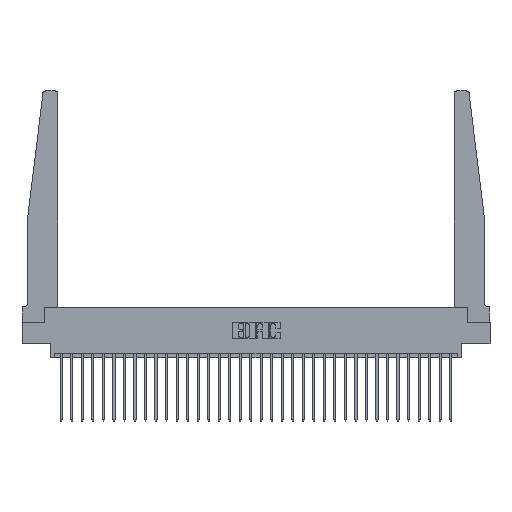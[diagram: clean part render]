
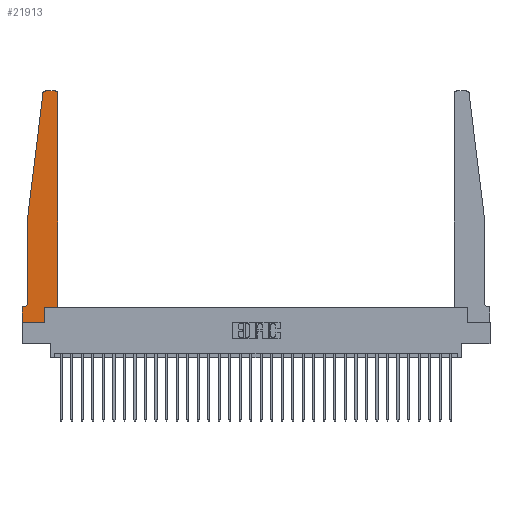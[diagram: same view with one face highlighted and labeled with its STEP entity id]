
A CAD part, top view. The second image highlights one B-rep face of the part: STEP entity #21913.
In plain terms, the highlighted planar face has unit normal (0, 0, 1).
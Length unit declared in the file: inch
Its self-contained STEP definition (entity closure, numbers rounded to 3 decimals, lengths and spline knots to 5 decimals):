
#366 = VERTEX_POINT ( 'NONE', #1723 ) ;
#1034 = CARTESIAN_POINT ( 'NONE',  ( 0., 0.1875, 0.37 ) ) ;
#1373 = CARTESIAN_POINT ( 'NONE',  ( 0.065, 1.25, 0.37 ) ) ;
#1605 = CIRCLE ( 'NONE', #3086, 0.03 ) ;
#1723 = CARTESIAN_POINT ( 'NONE',  ( 0.425, 0.18, 0.37 ) ) ;
#1725 = DIRECTION ( 'NONE',  ( 1., 0., 0. ) ) ;
#2872 = VECTOR ( 'NONE', #21808, 39.37008 ) ;
#3086 = AXIS2_PLACEMENT_3D ( 'NONE', #14151, #6574, #16016 ) ;
#3531 = CARTESIAN_POINT ( 'NONE',  ( 0.065, 0.2375, 0.37 ) ) ;
#3597 = LINE ( 'NONE', #22865, #25489 ) ;
#4220 = PLANE ( 'NONE',  #10039 ) ;
#4689 = ORIENTED_EDGE ( 'NONE', *, *, #11443, .T. ) ;
#4782 = DIRECTION ( 'NONE',  ( 1., 0., 0. ) ) ;
#4898 = VERTEX_POINT ( 'NONE', #26159 ) ;
#5219 = ORIENTED_EDGE ( 'NONE', *, *, #22220, .T. ) ;
#5363 = EDGE_CURVE ( 'NONE', #16599, #17011, #26127, .T. ) ;
#6184 = CARTESIAN_POINT ( 'NONE',  ( 0.2605, 0., 0.37 ) ) ;
#6529 = ORIENTED_EDGE ( 'NONE', *, *, #5363, .T. ) ;
#6574 = DIRECTION ( 'NONE',  ( 0., 0., 1. ) ) ;
#6626 = AXIS2_PLACEMENT_3D ( 'NONE', #6790, #25408, #11441 ) ;
#6790 = CARTESIAN_POINT ( 'NONE',  ( 0.395, 2.72, 0.37 ) ) ;
#7176 = FACE_OUTER_BOUND ( 'NONE', #26175, .T. ) ;
#7328 = ORIENTED_EDGE ( 'NONE', *, *, #22487, .T. ) ;
#7543 = VERTEX_POINT ( 'NONE', #1034 ) ;
#7659 = VERTEX_POINT ( 'NONE', #11002 ) ;
#8136 = DIRECTION ( 'NONE',  ( 1., 0., 0. ) ) ;
#8534 = AXIS2_PLACEMENT_3D ( 'NONE', #16651, #12298, #11993 ) ;
#8873 = CARTESIAN_POINT ( 'NONE',  ( 0.065, 0.1875, 0.37 ) ) ;
#9303 = CARTESIAN_POINT ( 'NONE',  ( 0., 0., 0.37 ) ) ;
#9388 = LINE ( 'NONE', #14193, #26004 ) ;
#10039 = AXIS2_PLACEMENT_3D ( 'NONE', #25802, #28436, #1725 ) ;
#10370 = EDGE_CURVE ( 'NONE', #29051, #27707, #21231, .T. ) ;
#10656 = VECTOR ( 'NONE', #8136, 39.37008 ) ;
#10984 = ORIENTED_EDGE ( 'NONE', *, *, #21948, .T. ) ;
#11002 = CARTESIAN_POINT ( 'NONE',  ( 0.425, 2.72, 0.37 ) ) ;
#11131 = ORIENTED_EDGE ( 'NONE', *, *, #14637, .T. ) ;
#11365 = DIRECTION ( 'NONE',  ( 0., 1., 0. ) ) ;
#11441 = DIRECTION ( 'NONE',  ( 1., 0., 0. ) ) ;
#11443 = EDGE_CURVE ( 'NONE', #4898, #7543, #30122, .T. ) ;
#11993 = DIRECTION ( 'NONE',  ( -1., 0., 0. ) ) ;
#12298 = DIRECTION ( 'NONE',  ( 0., 0., -1. ) ) ;
#13235 = VERTEX_POINT ( 'NONE', #15833 ) ;
#13278 = VERTEX_POINT ( 'NONE', #13818 ) ;
#13818 = CARTESIAN_POINT ( 'NONE',  ( 0.395, 2.75, 0.37 ) ) ;
#14151 = CARTESIAN_POINT ( 'NONE',  ( 0.27653, 2.72, 0.37 ) ) ;
#14171 = VECTOR ( 'NONE', #16279, 39.37008 ) ;
#14193 = CARTESIAN_POINT ( 'NONE',  ( 0., 0., 0.37 ) ) ;
#14201 = VERTEX_POINT ( 'NONE', #15314 ) ;
#14637 = EDGE_CURVE ( 'NONE', #13278, #14201, #29097, .T. ) ;
#15314 = CARTESIAN_POINT ( 'NONE',  ( 0.27653, 2.75, 0.37 ) ) ;
#15833 = CARTESIAN_POINT ( 'NONE',  ( 0.2605, 0.18, 0.37 ) ) ;
#16016 = DIRECTION ( 'NONE',  ( 1., 0., 0. ) ) ;
#16279 = DIRECTION ( 'NONE',  ( -1., 0., 0. ) ) ;
#16461 = EDGE_CURVE ( 'NONE', #366, #7659, #20522, .T. ) ;
#16599 = VERTEX_POINT ( 'NONE', #28285 ) ;
#16651 = CARTESIAN_POINT ( 'NONE',  ( 0.015, 0.2375, 0.37 ) ) ;
#17011 = VERTEX_POINT ( 'NONE', #23281 ) ;
#17697 = LINE ( 'NONE', #1373, #19509 ) ;
#17995 = CIRCLE ( 'NONE', #6626, 0.03 ) ;
#18149 = DIRECTION ( 'NONE',  ( -0.122, -0.992, 0. ) ) ;
#19509 = VECTOR ( 'NONE', #29655, 39.37008 ) ;
#20297 = EDGE_CURVE ( 'NONE', #28597, #4898, #22892, .T. ) ;
#20522 = LINE ( 'NONE', #22244, #23775 ) ;
#21231 = LINE ( 'NONE', #9303, #23056 ) ;
#21330 = ORIENTED_EDGE ( 'NONE', *, *, #27916, .T. ) ;
#21449 = ORIENTED_EDGE ( 'NONE', *, *, #23443, .T. ) ;
#21808 = DIRECTION ( 'NONE',  ( -1., 0., 0. ) ) ;
#21913 = ADVANCED_FACE ( 'NONE', ( #7176 ), #4220, .T. ) ;
#21948 = EDGE_CURVE ( 'NONE', #14201, #16599, #1605, .T. ) ;
#22132 = CARTESIAN_POINT ( 'NONE',  ( 0., 0., 0.37 ) ) ;
#22220 = EDGE_CURVE ( 'NONE', #17011, #28597, #17697, .T. ) ;
#22244 = CARTESIAN_POINT ( 'NONE',  ( 0.425, 0.18, 0.37 ) ) ;
#22487 = EDGE_CURVE ( 'NONE', #7659, #13278, #17995, .T. ) ;
#22553 = LINE ( 'NONE', #23979, #10656 ) ;
#22865 = CARTESIAN_POINT ( 'NONE',  ( 0.2605, 0.18, 0.37 ) ) ;
#22892 = CIRCLE ( 'NONE', #8534, 0.05 ) ;
#23056 = VECTOR ( 'NONE', #4782, 39.37008 ) ;
#23281 = CARTESIAN_POINT ( 'NONE',  ( 0.065, 1.25, 0.37 ) ) ;
#23443 = EDGE_CURVE ( 'NONE', #27707, #13235, #3597, .T. ) ;
#23775 = VECTOR ( 'NONE', #25033, 39.37008 ) ;
#23782 = VECTOR ( 'NONE', #18149, 39.37008 ) ;
#23979 = CARTESIAN_POINT ( 'NONE',  ( 0.425, 0.18, 0.37 ) ) ;
#24609 = EDGE_CURVE ( 'NONE', #7543, #29051, #9388, .T. ) ;
#24757 = ORIENTED_EDGE ( 'NONE', *, *, #10370, .T. ) ;
#25033 = DIRECTION ( 'NONE',  ( 0., 1., 0. ) ) ;
#25408 = DIRECTION ( 'NONE',  ( 0., 0., 1. ) ) ;
#25489 = VECTOR ( 'NONE', #11365, 39.37008 ) ;
#25802 = CARTESIAN_POINT ( 'NONE',  ( 0., 0.1875, 0.37 ) ) ;
#26004 = VECTOR ( 'NONE', #28322, 39.37008 ) ;
#26127 = LINE ( 'NONE', #27627, #23782 ) ;
#26159 = CARTESIAN_POINT ( 'NONE',  ( 0.015, 0.1875, 0.37 ) ) ;
#26175 = EDGE_LOOP ( 'NONE', ( #11131, #10984, #6529, #5219, #30046, #4689, #28590, #24757, #21449, #21330, #29842, #7328 ) ) ;
#26773 = CARTESIAN_POINT ( 'NONE',  ( 0.25, 2.75, 0.37 ) ) ;
#27627 = CARTESIAN_POINT ( 'NONE',  ( 0.065, 1.25, 0.37 ) ) ;
#27707 = VERTEX_POINT ( 'NONE', #6184 ) ;
#27916 = EDGE_CURVE ( 'NONE', #13235, #366, #22553, .T. ) ;
#28285 = CARTESIAN_POINT ( 'NONE',  ( 0.24675, 2.72367, 0.37 ) ) ;
#28322 = DIRECTION ( 'NONE',  ( 0., -1., 0. ) ) ;
#28436 = DIRECTION ( 'NONE',  ( 0., 0., 1. ) ) ;
#28590 = ORIENTED_EDGE ( 'NONE', *, *, #24609, .T. ) ;
#28597 = VERTEX_POINT ( 'NONE', #3531 ) ;
#29051 = VERTEX_POINT ( 'NONE', #22132 ) ;
#29097 = LINE ( 'NONE', #26773, #2872 ) ;
#29655 = DIRECTION ( 'NONE',  ( 0., -1., 0. ) ) ;
#29842 = ORIENTED_EDGE ( 'NONE', *, *, #16461, .T. ) ;
#30046 = ORIENTED_EDGE ( 'NONE', *, *, #20297, .T. ) ;
#30122 = LINE ( 'NONE', #8873, #14171 ) ;
